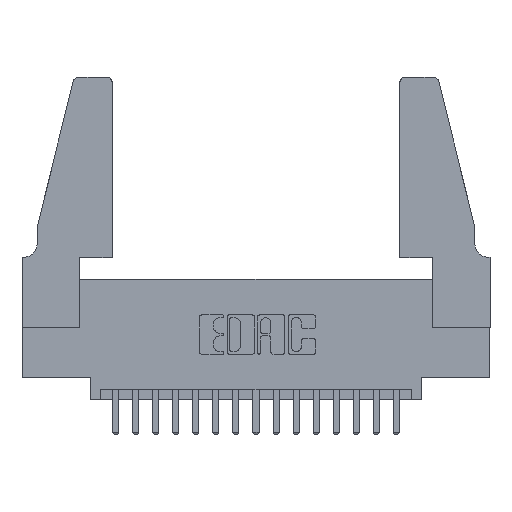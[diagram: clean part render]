
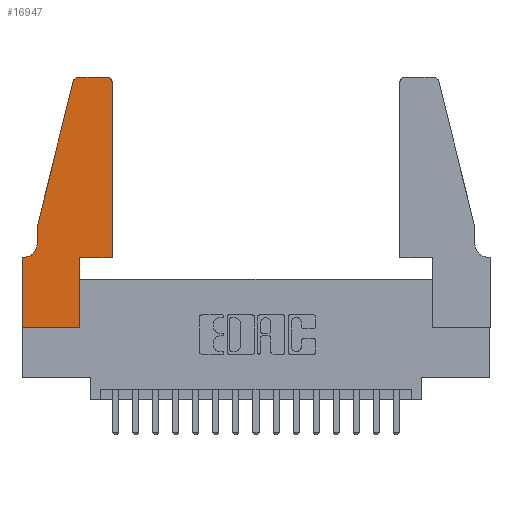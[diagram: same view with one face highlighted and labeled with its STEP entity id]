
A CAD part, top view. The second image highlights one B-rep face of the part: STEP entity #16947.
In plain terms, the highlighted planar face has unit normal (0, 0, 1).
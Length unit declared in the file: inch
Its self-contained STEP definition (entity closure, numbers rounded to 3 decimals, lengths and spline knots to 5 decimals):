
#147 = DIRECTION ( 'NONE',  ( -1., 0., 0. ) ) ;
#380 = DIRECTION ( 'NONE',  ( 0., 1., 0. ) ) ;
#383 = VERTEX_POINT ( 'NONE', #5630 ) ;
#509 = DIRECTION ( 'NONE',  ( 0., 0., -1. ) ) ;
#595 = VECTOR ( 'NONE', #1048, 39.37008 ) ;
#647 = CARTESIAN_POINT ( 'NONE',  ( 0.2865, 0.35, 0.37 ) ) ;
#649 = VECTOR ( 'NONE', #3743, 39.37008 ) ;
#986 = CARTESIAN_POINT ( 'NONE',  ( 0., 0., 0.37 ) ) ;
#1048 = DIRECTION ( 'NONE',  ( -0.239, -0.971, 0. ) ) ;
#1076 = CIRCLE ( 'NONE', #2963, 0.03 ) ;
#1251 = CARTESIAN_POINT ( 'NONE',  ( 0.284, 1.25, 0.37 ) ) ;
#1744 = ORIENTED_EDGE ( 'NONE', *, *, #10902, .T. ) ;
#2229 = CIRCLE ( 'NONE', #7860, 0.07 ) ;
#2342 = VECTOR ( 'NONE', #11968, 39.37008 ) ;
#2374 = CARTESIAN_POINT ( 'NONE',  ( 0.0755, 0.5, 0.37 ) ) ;
#2401 = DIRECTION ( 'NONE',  ( 1., 0., 0. ) ) ;
#2423 = CARTESIAN_POINT ( 'NONE',  ( 0.0755, 0.5, 0.37 ) ) ;
#2462 = CARTESIAN_POINT ( 'NONE',  ( 0.0755, 0.5, 0.37 ) ) ;
#2698 = ORIENTED_EDGE ( 'NONE', *, *, #6300, .T. ) ;
#2963 = AXIS2_PLACEMENT_3D ( 'NONE', #10481, #7878, #7760 ) ;
#3128 = CARTESIAN_POINT ( 'NONE',  ( 0.0055, 0.42, 0.37 ) ) ;
#3344 = ORIENTED_EDGE ( 'NONE', *, *, #11779, .T. ) ;
#3371 = VERTEX_POINT ( 'NONE', #15307 ) ;
#3743 = DIRECTION ( 'NONE',  ( 0., -1., 0. ) ) ;
#4058 = VECTOR ( 'NONE', #147, 39.37008 ) ;
#4115 = ORIENTED_EDGE ( 'NONE', *, *, #17669, .T. ) ;
#4212 = EDGE_CURVE ( 'NONE', #14806, #15425, #15930, .T. ) ;
#4747 = FACE_OUTER_BOUND ( 'NONE', #15794, .T. ) ;
#4905 = CARTESIAN_POINT ( 'NONE',  ( 0.0755, 0.42, 0.37 ) ) ;
#5630 = CARTESIAN_POINT ( 'NONE',  ( 0.4205, 1.25, 0.37 ) ) ;
#5666 = CARTESIAN_POINT ( 'NONE',  ( 0.2865, 0.35, 0.37 ) ) ;
#6300 = EDGE_CURVE ( 'NONE', #11046, #14806, #7876, .T. ) ;
#6303 = EDGE_CURVE ( 'NONE', #11915, #14891, #9596, .T. ) ;
#6323 = ORIENTED_EDGE ( 'NONE', *, *, #13172, .T. ) ;
#6334 = CARTESIAN_POINT ( 'NONE',  ( 0.4205, 1.22, 0.37 ) ) ;
#6579 = CARTESIAN_POINT ( 'NONE',  ( 0.4505, 0.35, 0.37 ) ) ;
#7179 = VECTOR ( 'NONE', #9793, 39.37008 ) ;
#7760 = DIRECTION ( 'NONE',  ( 1., 0., 0. ) ) ;
#7830 = DIRECTION ( 'NONE',  ( 1., 0., 0. ) ) ;
#7860 = AXIS2_PLACEMENT_3D ( 'NONE', #3128, #509, #15534 ) ;
#7876 = LINE ( 'NONE', #2462, #595 ) ;
#7878 = DIRECTION ( 'NONE',  ( 0., 0., 1. ) ) ;
#7927 = ORIENTED_EDGE ( 'NONE', *, *, #12244, .T. ) ;
#7951 = EDGE_CURVE ( 'NONE', #15425, #3371, #2229, .T. ) ;
#8013 = LINE ( 'NONE', #12467, #7179 ) ;
#8210 = VECTOR ( 'NONE', #15901, 39.37008 ) ;
#8241 = DIRECTION ( 'NONE',  ( 1., 0., 0. ) ) ;
#8287 = CARTESIAN_POINT ( 'NONE',  ( 0.0755, 0.35, 0.37 ) ) ;
#8614 = VECTOR ( 'NONE', #380, 39.37008 ) ;
#8907 = VERTEX_POINT ( 'NONE', #1251 ) ;
#9503 = PLANE ( 'NONE',  #16223 ) ;
#9596 = LINE ( 'NONE', #16186, #17801 ) ;
#9696 = CARTESIAN_POINT ( 'NONE',  ( 0.4505, 1.22, 0.37 ) ) ;
#9703 = LINE ( 'NONE', #13048, #8210 ) ;
#9793 = DIRECTION ( 'NONE',  ( 0., 1., 0. ) ) ;
#9794 = CARTESIAN_POINT ( 'NONE',  ( 0.4505, 0.35, 0.37 ) ) ;
#10417 = CIRCLE ( 'NONE', #10660, 0.03 ) ;
#10481 = CARTESIAN_POINT ( 'NONE',  ( 0.284, 1.22, 0.37 ) ) ;
#10541 = EDGE_CURVE ( 'NONE', #16273, #383, #10417, .T. ) ;
#10660 = AXIS2_PLACEMENT_3D ( 'NONE', #6334, #17420, #7830 ) ;
#10711 = ORIENTED_EDGE ( 'NONE', *, *, #11870, .T. ) ;
#10838 = DIRECTION ( 'NONE',  ( 0., 0., 1. ) ) ;
#10846 = CARTESIAN_POINT ( 'NONE',  ( 0.2865, 0., 0.37 ) ) ;
#10902 = EDGE_CURVE ( 'NONE', #13569, #16273, #8013, .T. ) ;
#11046 = VERTEX_POINT ( 'NONE', #13112 ) ;
#11181 = ORIENTED_EDGE ( 'NONE', *, *, #17358, .T. ) ;
#11226 = VECTOR ( 'NONE', #14385, 39.37008 ) ;
#11779 = EDGE_CURVE ( 'NONE', #383, #8907, #9703, .T. ) ;
#11870 = EDGE_CURVE ( 'NONE', #13905, #11915, #15968, .T. ) ;
#11915 = VERTEX_POINT ( 'NONE', #986 ) ;
#11968 = DIRECTION ( 'NONE',  ( 1., 0., 0. ) ) ;
#11981 = LINE ( 'NONE', #8287, #4058 ) ;
#12244 = EDGE_CURVE ( 'NONE', #14891, #15214, #12263, .T. ) ;
#12263 = LINE ( 'NONE', #5666, #8614 ) ;
#12404 = CARTESIAN_POINT ( 'NONE',  ( 0., 0.35, 0.37 ) ) ;
#12467 = CARTESIAN_POINT ( 'NONE',  ( 0.4505, 0.35, 0.37 ) ) ;
#12670 = LINE ( 'NONE', #6579, #2342 ) ;
#12805 = ORIENTED_EDGE ( 'NONE', *, *, #7951, .T. ) ;
#13048 = CARTESIAN_POINT ( 'NONE',  ( 0.2605, 1.25, 0.37 ) ) ;
#13082 = ORIENTED_EDGE ( 'NONE', *, *, #4212, .T. ) ;
#13112 = CARTESIAN_POINT ( 'NONE',  ( 0.25487, 1.22718, 0.37 ) ) ;
#13172 = EDGE_CURVE ( 'NONE', #15214, #13569, #12670, .T. ) ;
#13525 = CARTESIAN_POINT ( 'NONE',  ( 0., 0.35, 0.37 ) ) ;
#13569 = VERTEX_POINT ( 'NONE', #9794 ) ;
#13905 = VERTEX_POINT ( 'NONE', #13525 ) ;
#14385 = DIRECTION ( 'NONE',  ( 0., -1., 0. ) ) ;
#14806 = VERTEX_POINT ( 'NONE', #2374 ) ;
#14891 = VERTEX_POINT ( 'NONE', #10846 ) ;
#15214 = VERTEX_POINT ( 'NONE', #647 ) ;
#15307 = CARTESIAN_POINT ( 'NONE',  ( 0.0055, 0.35, 0.37 ) ) ;
#15425 = VERTEX_POINT ( 'NONE', #4905 ) ;
#15534 = DIRECTION ( 'NONE',  ( -1., 0., 0. ) ) ;
#15585 = ORIENTED_EDGE ( 'NONE', *, *, #10541, .T. ) ;
#15794 = EDGE_LOOP ( 'NONE', ( #3344, #11181, #2698, #13082, #12805, #4115, #10711, #16765, #7927, #6323, #1744, #15585 ) ) ;
#15901 = DIRECTION ( 'NONE',  ( -1., 0., 0. ) ) ;
#15930 = LINE ( 'NONE', #2423, #649 ) ;
#15968 = LINE ( 'NONE', #17277, #11226 ) ;
#16186 = CARTESIAN_POINT ( 'NONE',  ( 0., 0., 0.37 ) ) ;
#16223 = AXIS2_PLACEMENT_3D ( 'NONE', #12404, #10838, #8241 ) ;
#16273 = VERTEX_POINT ( 'NONE', #9696 ) ;
#16765 = ORIENTED_EDGE ( 'NONE', *, *, #6303, .T. ) ;
#16947 = ADVANCED_FACE ( 'NONE', ( #4747 ), #9503, .T. ) ;
#17277 = CARTESIAN_POINT ( 'NONE',  ( 0., 0., 0.37 ) ) ;
#17358 = EDGE_CURVE ( 'NONE', #8907, #11046, #1076, .T. ) ;
#17420 = DIRECTION ( 'NONE',  ( 0., 0., 1. ) ) ;
#17669 = EDGE_CURVE ( 'NONE', #3371, #13905, #11981, .T. ) ;
#17801 = VECTOR ( 'NONE', #2401, 39.37008 ) ;
